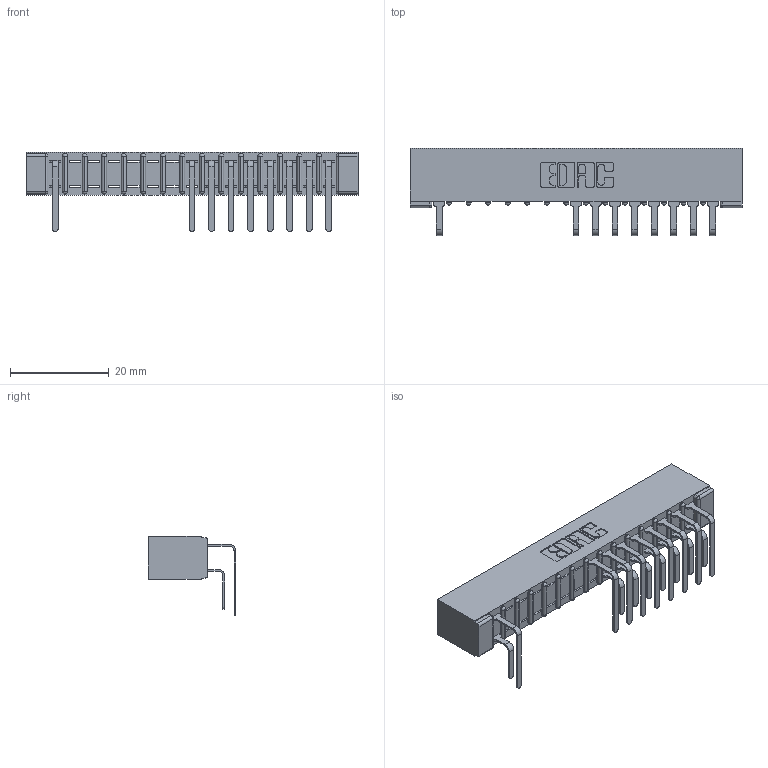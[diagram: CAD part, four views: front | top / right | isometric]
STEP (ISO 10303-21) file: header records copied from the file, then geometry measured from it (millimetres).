
FILE_DESCRIPTION (( 'STEP AP203' ), '1' );
FILE_NAME ('307-030-559-201.STEP', '2018-08-04T19:55:07', ( '' ), ( '' ), 'SwSTEP 2.0', 'SolidWorks 2016', '' );
FILE_SCHEMA (( 'CONFIG_CONTROL_DESIGN' ));
Length unit declared in the file: inch
Products named in the file (4): 307 Part_No Mounting Lugs; 307-290-001_558 559 - 1 (Single); 307-290-001_559 - 2 (Single); 307-030-559-201
Assembly tree (18 placements, depth 2):
  307-030-559-201
    307 Part_No Mounting Lugs
    307-290-001_558 559 - 1 (Single)  x8
    307-290-001_559 - 2 (Single)  x9
Bounding box: 67.31 x 17.69 x 16.08 mm (x, y, z)
Volume: 4545.4 mm3; surface area: 7574.1 mm2
Topology: 18 solids, 18 shells, 1106 faces, 3129 edges, 2018 vertices
Faces by surface type: plane 705, cylinder 369, sphere 32
Entity records: 17421 total; most frequent: CARTESIAN_POINT 2912, ORIENTED_EDGE 2894, DIRECTION 2849, EDGE_CURVE 1447, LINE 1099, VECTOR 1099, VERTEX_POINT 938, AXIS2_PLACEMENT_3D 875
